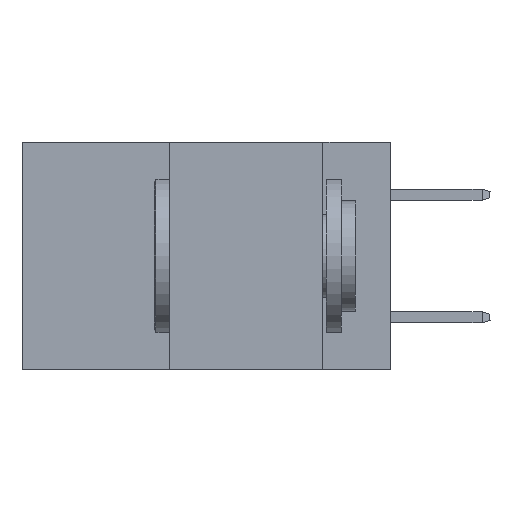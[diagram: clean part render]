
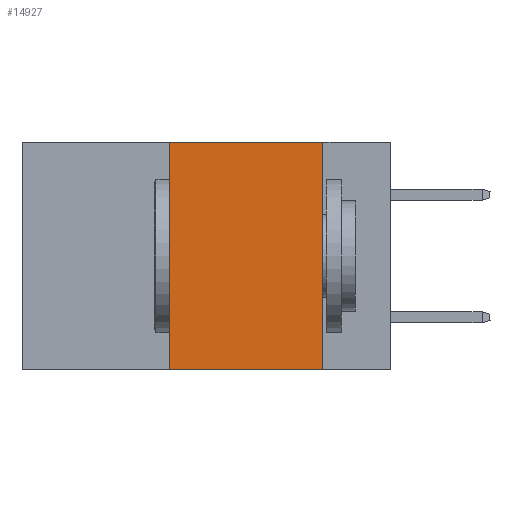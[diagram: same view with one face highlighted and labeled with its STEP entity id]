
A CAD part, left-side view. The second image highlights one B-rep face of the part: STEP entity #14927.
In plain terms, the highlighted planar face has unit normal (-1, 0, 0).
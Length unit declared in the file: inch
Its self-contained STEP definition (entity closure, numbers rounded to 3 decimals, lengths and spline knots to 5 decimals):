
#935 = LINE ( 'NONE', #4699, #1735 ) ;
#1391 = CARTESIAN_POINT ( 'NONE',  ( 0., 0.6, 0. ) ) ;
#1735 = VECTOR ( 'NONE', #14856, 39.37008 ) ;
#2281 = VECTOR ( 'NONE', #9325, 39.37008 ) ;
#2330 = EDGE_LOOP ( 'NONE', ( #9532, #11309, #9396, #8101 ) ) ;
#2480 = VECTOR ( 'NONE', #9529, 39.37008 ) ;
#3125 = VERTEX_POINT ( 'NONE', #4080 ) ;
#3725 = FACE_OUTER_BOUND ( 'NONE', #2330, .T. ) ;
#4080 = CARTESIAN_POINT ( 'NONE',  ( 0., 0.11, 0. ) ) ;
#4198 = CARTESIAN_POINT ( 'NONE',  ( 0., 0.36, 0. ) ) ;
#4534 = CARTESIAN_POINT ( 'NONE',  ( 0., 0.36, 0. ) ) ;
#4699 = CARTESIAN_POINT ( 'NONE',  ( 0., 0.11, 0. ) ) ;
#4835 = PLANE ( 'NONE',  #7167 ) ;
#7167 = AXIS2_PLACEMENT_3D ( 'NONE', #12408, #7364, #7529 ) ;
#7364 = DIRECTION ( 'NONE',  ( 1., 0., 0. ) ) ;
#7529 = DIRECTION ( 'NONE',  ( 0., 0., -1. ) ) ;
#7670 = EDGE_CURVE ( 'NONE', #3125, #13775, #935, .T. ) ;
#8078 = CARTESIAN_POINT ( 'NONE',  ( 0., 0.6, -0.37 ) ) ;
#8101 = ORIENTED_EDGE ( 'NONE', *, *, #8816, .T. ) ;
#8816 = EDGE_CURVE ( 'NONE', #12933, #13775, #11134, .T. ) ;
#9025 = DIRECTION ( 'NONE',  ( 0., -1., 0. ) ) ;
#9245 = LINE ( 'NONE', #1391, #11001 ) ;
#9280 = EDGE_CURVE ( 'NONE', #12933, #15847, #13073, .T. ) ;
#9325 = DIRECTION ( 'NONE',  ( 0., -1., 0. ) ) ;
#9396 = ORIENTED_EDGE ( 'NONE', *, *, #9280, .F. ) ;
#9529 = DIRECTION ( 'NONE',  ( 0., 0., 1. ) ) ;
#9532 = ORIENTED_EDGE ( 'NONE', *, *, #7670, .F. ) ;
#11001 = VECTOR ( 'NONE', #9025, 39.37008 ) ;
#11134 = LINE ( 'NONE', #8078, #2281 ) ;
#11309 = ORIENTED_EDGE ( 'NONE', *, *, #14282, .F. ) ;
#12408 = CARTESIAN_POINT ( 'NONE',  ( 0., 0.6, 0. ) ) ;
#12573 = CARTESIAN_POINT ( 'NONE',  ( 0., 0.36, -0.37 ) ) ;
#12872 = CARTESIAN_POINT ( 'NONE',  ( 0., 0.11, -0.37 ) ) ;
#12933 = VERTEX_POINT ( 'NONE', #12573 ) ;
#13073 = LINE ( 'NONE', #4534, #2480 ) ;
#13775 = VERTEX_POINT ( 'NONE', #12872 ) ;
#14282 = EDGE_CURVE ( 'NONE', #15847, #3125, #9245, .T. ) ;
#14856 = DIRECTION ( 'NONE',  ( 0., 0., -1. ) ) ;
#14927 = ADVANCED_FACE ( 'NONE', ( #3725 ), #4835, .F. ) ;
#15847 = VERTEX_POINT ( 'NONE', #4198 ) ;
